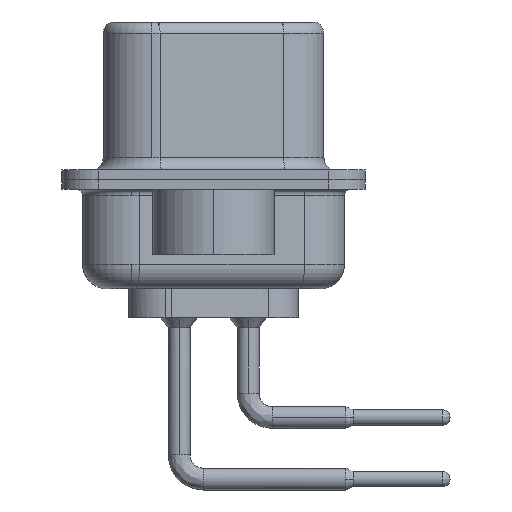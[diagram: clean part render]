
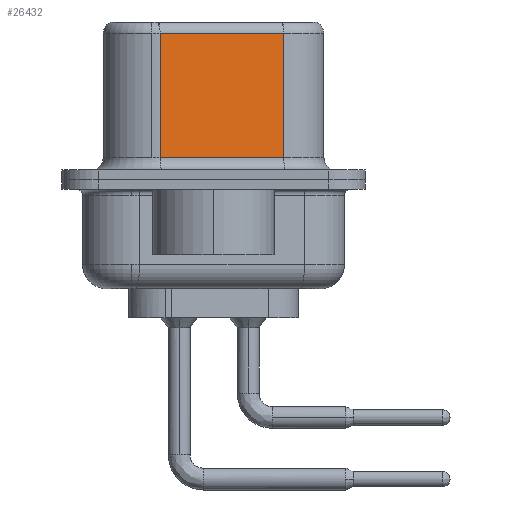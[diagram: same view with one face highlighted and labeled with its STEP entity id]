
A CAD part, left-side view. The second image highlights one B-rep face of the part: STEP entity #26432.
In plain terms, the highlighted planar face has unit normal (-0.985, -0.174, 0).
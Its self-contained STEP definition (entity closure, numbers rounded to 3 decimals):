
#476 = CARTESIAN_POINT ( 'NONE',  ( 4.58, -2.897, 0.9 ) ) ;
#790 = EDGE_CURVE ( 'NONE', #13431, #23856, #21804, .T. ) ;
#815 = AXIS2_PLACEMENT_3D ( 'NONE', #7943, #26622, #12641 ) ;
#1037 = EDGE_CURVE ( 'NONE', #25552, #13431, #15979, .T. ) ;
#2027 = VECTOR ( 'NONE', #21898, 1000. ) ;
#2400 = EDGE_CURVE ( 'NONE', #8084, #23856, #19497, .T. ) ;
#3879 = CARTESIAN_POINT ( 'NONE',  ( 3.68, 2.203, 6.02 ) ) ;
#3927 = VECTOR ( 'NONE', #20565, 1000. ) ;
#5322 = CARTESIAN_POINT ( 'NONE',  ( 4.58, -2.897, 6.02 ) ) ;
#6301 = VECTOR ( 'NONE', #13953, 1000. ) ;
#7943 = CARTESIAN_POINT ( 'NONE',  ( 4.58, -2.897, 6.52 ) ) ;
#8084 = VERTEX_POINT ( 'NONE', #5322 ) ;
#8329 = ORIENTED_EDGE ( 'NONE', *, *, #1037, .T. ) ;
#11603 = CARTESIAN_POINT ( 'NONE',  ( 4.58, -2.897, 6.02 ) ) ;
#12641 = DIRECTION ( 'NONE',  ( -0.174, 0.985, 0. ) ) ;
#13431 = VERTEX_POINT ( 'NONE', #29298 ) ;
#13953 = DIRECTION ( 'NONE',  ( -0.174, 0.985, 0. ) ) ;
#15008 = ORIENTED_EDGE ( 'NONE', *, *, #790, .T. ) ;
#15979 = LINE ( 'NONE', #18278, #2027 ) ;
#16653 = FACE_OUTER_BOUND ( 'NONE', #22909, .T. ) ;
#17551 = ORIENTED_EDGE ( 'NONE', *, *, #28979, .T. ) ;
#18278 = CARTESIAN_POINT ( 'NONE',  ( 3.68, 2.203, 6.52 ) ) ;
#19497 = LINE ( 'NONE', #28189, #25002 ) ;
#20565 = DIRECTION ( 'NONE',  ( 0.174, -0.985, 0. ) ) ;
#20625 = ORIENTED_EDGE ( 'NONE', *, *, #2400, .F. ) ;
#21804 = LINE ( 'NONE', #30065, #3927 ) ;
#21898 = DIRECTION ( 'NONE',  ( 0., 0., -1. ) ) ;
#22909 = EDGE_LOOP ( 'NONE', ( #20625, #17551, #8329, #15008 ) ) ;
#23856 = VERTEX_POINT ( 'NONE', #476 ) ;
#24178 = LINE ( 'NONE', #11603, #6301 ) ;
#24232 = PLANE ( 'NONE',  #815 ) ;
#25002 = VECTOR ( 'NONE', #28431, 1000. ) ;
#25552 = VERTEX_POINT ( 'NONE', #3879 ) ;
#26432 = ADVANCED_FACE ( 'NONE', ( #16653 ), #24232, .F. ) ;
#26622 = DIRECTION ( 'NONE',  ( 0.985, 0.174, 0. ) ) ;
#28189 = CARTESIAN_POINT ( 'NONE',  ( 4.58, -2.897, 6.52 ) ) ;
#28431 = DIRECTION ( 'NONE',  ( 0., 0., -1. ) ) ;
#28979 = EDGE_CURVE ( 'NONE', #8084, #25552, #24178, .T. ) ;
#29298 = CARTESIAN_POINT ( 'NONE',  ( 3.68, 2.203, 0.9 ) ) ;
#30065 = CARTESIAN_POINT ( 'NONE',  ( 4.58, -2.897, 0.9 ) ) ;
